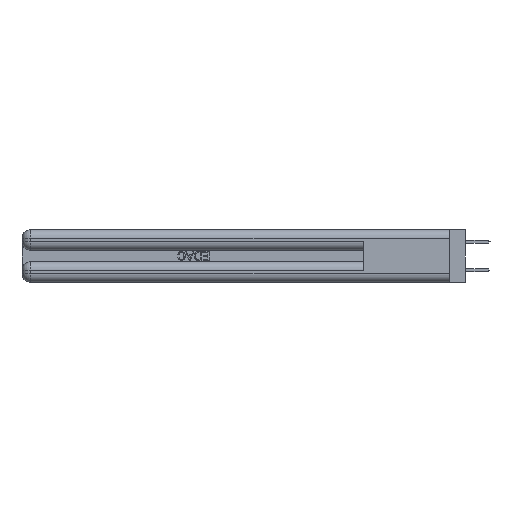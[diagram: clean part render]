
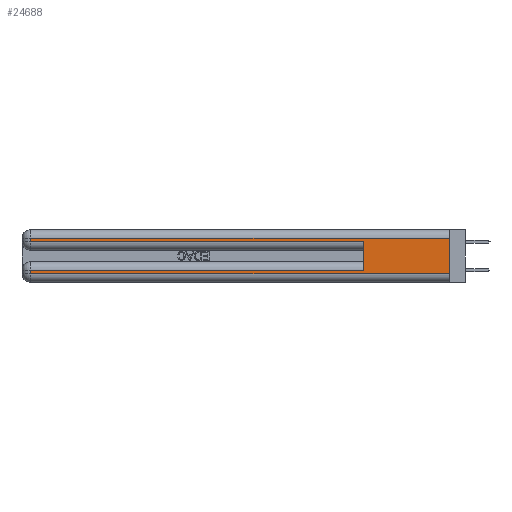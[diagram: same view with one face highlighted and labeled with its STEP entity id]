
A CAD part, left-side view. The second image highlights one B-rep face of the part: STEP entity #24688.
In plain terms, the highlighted planar face has unit normal (-1, 0, 0).
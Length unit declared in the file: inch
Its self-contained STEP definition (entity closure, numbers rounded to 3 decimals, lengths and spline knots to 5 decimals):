
#50 = DIRECTION ( 'NONE',  ( 0., 1., 0. ) ) ;
#291 = DIRECTION ( 'NONE',  ( 0., -1., 0. ) ) ;
#635 = DIRECTION ( 'NONE',  ( 0., 0., -1. ) ) ;
#855 = ORIENTED_EDGE ( 'NONE', *, *, #3592, .T. ) ;
#1881 = LINE ( 'NONE', #5180, #35095 ) ;
#2892 = LINE ( 'NONE', #19894, #19551 ) ;
#3592 = EDGE_CURVE ( 'NONE', #13184, #4411, #10886, .T. ) ;
#3893 = CARTESIAN_POINT ( 'NONE',  ( 0., 0., 0.06 ) ) ;
#4411 = VERTEX_POINT ( 'NONE', #3893 ) ;
#5180 = CARTESIAN_POINT ( 'NONE',  ( 0., 2.94, 0.37 ) ) ;
#5320 = CARTESIAN_POINT ( 'NONE',  ( 0., 0.6, 0.285 ) ) ;
#5917 = DIRECTION ( 'NONE',  ( 0., -1., 0. ) ) ;
#6845 = VECTOR ( 'NONE', #40978, 39.37008 ) ;
#7560 = LINE ( 'NONE', #24219, #32208 ) ;
#7861 = LINE ( 'NONE', #34502, #6845 ) ;
#8048 = ORIENTED_EDGE ( 'NONE', *, *, #8239, .F. ) ;
#8239 = EDGE_CURVE ( 'NONE', #26194, #10807, #7560, .T. ) ;
#8611 = CARTESIAN_POINT ( 'NONE',  ( 0., 0., 0.31 ) ) ;
#9365 = ORIENTED_EDGE ( 'NONE', *, *, #25019, .T. ) ;
#10216 = VECTOR ( 'NONE', #50, 39.37008 ) ;
#10765 = EDGE_CURVE ( 'NONE', #38260, #13184, #1881, .T. ) ;
#10807 = VERTEX_POINT ( 'NONE', #5320 ) ;
#10886 = LINE ( 'NONE', #25200, #28027 ) ;
#11227 = DIRECTION ( 'NONE',  ( 0., 0., 1. ) ) ;
#11283 = DIRECTION ( 'NONE',  ( 1., 0., 0. ) ) ;
#11494 = EDGE_CURVE ( 'NONE', #26194, #38260, #7861, .T. ) ;
#13184 = VERTEX_POINT ( 'NONE', #23722 ) ;
#13332 = VECTOR ( 'NONE', #15162, 39.37008 ) ;
#13991 = EDGE_LOOP ( 'NONE', ( #28162, #9365, #39037, #40927, #8048, #21232, #14408, #855 ) ) ;
#14408 = ORIENTED_EDGE ( 'NONE', *, *, #10765, .T. ) ;
#15162 = DIRECTION ( 'NONE',  ( 0., 0., -1. ) ) ;
#15373 = LINE ( 'NONE', #24766, #13332 ) ;
#15846 = CARTESIAN_POINT ( 'NONE',  ( 0., 0.6, 0.085 ) ) ;
#18788 = LINE ( 'NONE', #35755, #10216 ) ;
#19551 = VECTOR ( 'NONE', #635, 39.37008 ) ;
#19751 = EDGE_CURVE ( 'NONE', #37245, #10807, #38290, .T. ) ;
#19894 = CARTESIAN_POINT ( 'NONE',  ( 0., 2.94, 0.37 ) ) ;
#20741 = VERTEX_POINT ( 'NONE', #8611 ) ;
#21232 = ORIENTED_EDGE ( 'NONE', *, *, #11494, .T. ) ;
#22097 = CARTESIAN_POINT ( 'NONE',  ( 0., 2.94, 0.285 ) ) ;
#22106 = EDGE_CURVE ( 'NONE', #40473, #37245, #2892, .T. ) ;
#23580 = EDGE_CURVE ( 'NONE', #20741, #4411, #15373, .T. ) ;
#23722 = CARTESIAN_POINT ( 'NONE',  ( 0., 2.94, 0.06 ) ) ;
#24128 = PLANE ( 'NONE',  #35419 ) ;
#24219 = CARTESIAN_POINT ( 'NONE',  ( 0., 0.6, 0.145 ) ) ;
#24447 = DIRECTION ( 'NONE',  ( 0., 0., -1. ) ) ;
#24688 = ADVANCED_FACE ( 'NONE', ( #38415 ), #24128, .F. ) ;
#24766 = CARTESIAN_POINT ( 'NONE',  ( 0., 0., 0.37 ) ) ;
#25019 = EDGE_CURVE ( 'NONE', #20741, #40473, #18788, .T. ) ;
#25200 = CARTESIAN_POINT ( 'NONE',  ( 0., 0., 0.06 ) ) ;
#26194 = VERTEX_POINT ( 'NONE', #15846 ) ;
#26238 = CARTESIAN_POINT ( 'NONE',  ( 0., 2.94, 0.085 ) ) ;
#28027 = VECTOR ( 'NONE', #5917, 39.37008 ) ;
#28162 = ORIENTED_EDGE ( 'NONE', *, *, #23580, .F. ) ;
#29743 = VECTOR ( 'NONE', #291, 39.37008 ) ;
#30568 = CARTESIAN_POINT ( 'NONE',  ( 0., 0., 0.37 ) ) ;
#30663 = CARTESIAN_POINT ( 'NONE',  ( 0., 2.94, 0.31 ) ) ;
#32208 = VECTOR ( 'NONE', #11227, 39.37008 ) ;
#33792 = DIRECTION ( 'NONE',  ( 0., 0., -1. ) ) ;
#34502 = CARTESIAN_POINT ( 'NONE',  ( 0., 0., 0.085 ) ) ;
#35095 = VECTOR ( 'NONE', #24447, 39.37008 ) ;
#35419 = AXIS2_PLACEMENT_3D ( 'NONE', #30568, #11283, #33792 ) ;
#35755 = CARTESIAN_POINT ( 'NONE',  ( 0., 0., 0.31 ) ) ;
#37245 = VERTEX_POINT ( 'NONE', #22097 ) ;
#38260 = VERTEX_POINT ( 'NONE', #26238 ) ;
#38290 = LINE ( 'NONE', #38795, #29743 ) ;
#38415 = FACE_OUTER_BOUND ( 'NONE', #13991, .T. ) ;
#38795 = CARTESIAN_POINT ( 'NONE',  ( 0., 0., 0.285 ) ) ;
#39037 = ORIENTED_EDGE ( 'NONE', *, *, #22106, .T. ) ;
#40473 = VERTEX_POINT ( 'NONE', #30663 ) ;
#40927 = ORIENTED_EDGE ( 'NONE', *, *, #19751, .T. ) ;
#40978 = DIRECTION ( 'NONE',  ( 0., 1., 0. ) ) ;
